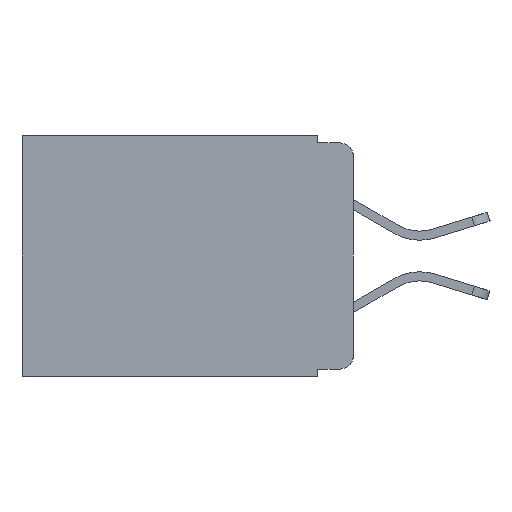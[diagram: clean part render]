
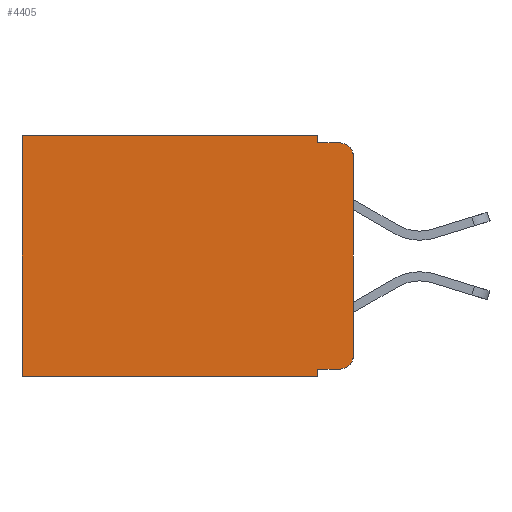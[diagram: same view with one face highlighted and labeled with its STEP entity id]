
A CAD part, left-side view. The second image highlights one B-rep face of the part: STEP entity #4405.
In plain terms, the highlighted planar face has unit normal (-1, 0, 0).
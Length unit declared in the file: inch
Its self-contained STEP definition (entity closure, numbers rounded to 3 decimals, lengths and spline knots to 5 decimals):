
#244 = VECTOR ( 'NONE', #6676, 39.37008 ) ;
#445 = VECTOR ( 'NONE', #9606, 39.37008 ) ;
#461 = ORIENTED_EDGE ( 'NONE', *, *, #2379, .T. ) ;
#706 = EDGE_LOOP ( 'NONE', ( #2293, #2764, #3546, #811, #461, #4432, #4359, #2546, #3100, #4057 ) ) ;
#811 = ORIENTED_EDGE ( 'NONE', *, *, #1928, .F. ) ;
#1293 = EDGE_CURVE ( 'NONE', #8706, #2113, #6968, .T. ) ;
#1497 = LINE ( 'NONE', #3207, #8030 ) ;
#1835 = EDGE_CURVE ( 'NONE', #3333, #5252, #5842, .T. ) ;
#1911 = EDGE_CURVE ( 'NONE', #3333, #3045, #3982, .T. ) ;
#1913 = EDGE_CURVE ( 'NONE', #5400, #3045, #1497, .T. ) ;
#1928 = EDGE_CURVE ( 'NONE', #6808, #5400, #9977, .T. ) ;
#1972 = EDGE_CURVE ( 'NONE', #2336, #2113, #5190, .T. ) ;
#1988 = EDGE_CURVE ( 'NONE', #3810, #8706, #2867, .T. ) ;
#2025 = EDGE_CURVE ( 'NONE', #3810, #10645, #6342, .T. ) ;
#2074 = EDGE_CURVE ( 'NONE', #10645, #5252, #3568, .T. ) ;
#2103 = CARTESIAN_POINT ( 'NONE',  ( 0.298, 0.051, -0.343 ) ) ;
#2113 = VERTEX_POINT ( 'NONE', #9554 ) ;
#2293 = ORIENTED_EDGE ( 'NONE', *, *, #1835, .F. ) ;
#2336 = VERTEX_POINT ( 'NONE', #8853 ) ;
#2379 = EDGE_CURVE ( 'NONE', #6808, #2336, #9163, .T. ) ;
#2443 = DIRECTION ( 'NONE',  ( -1., 0., 0. ) ) ;
#2546 = ORIENTED_EDGE ( 'NONE', *, *, #1988, .F. ) ;
#2573 = CARTESIAN_POINT ( 'NONE',  ( 0.298, 0.02, -0.313 ) ) ;
#2764 = ORIENTED_EDGE ( 'NONE', *, *, #1911, .T. ) ;
#2867 = LINE ( 'NONE', #8884, #7063 ) ;
#2917 = FACE_OUTER_BOUND ( 'NONE', #706, .T. ) ;
#3023 = CARTESIAN_POINT ( 'NONE',  ( 0.298, 0., 0. ) ) ;
#3045 = VERTEX_POINT ( 'NONE', #4628 ) ;
#3067 = CARTESIAN_POINT ( 'NONE',  ( 0.298, 0.02, -0.03 ) ) ;
#3100 = ORIENTED_EDGE ( 'NONE', *, *, #2025, .T. ) ;
#3207 = CARTESIAN_POINT ( 'NONE',  ( 0.298, 0.051, -0.01 ) ) ;
#3281 = VECTOR ( 'NONE', #9714, 39.37008 ) ;
#3333 = VERTEX_POINT ( 'NONE', #9575 ) ;
#3546 = ORIENTED_EDGE ( 'NONE', *, *, #1913, .F. ) ;
#3568 = CIRCLE ( 'NONE', #4679, 0.02 ) ;
#3810 = VERTEX_POINT ( 'NONE', #9074 ) ;
#3931 = CARTESIAN_POINT ( 'NONE',  ( 0.298, 0.051, 0. ) ) ;
#3982 = CIRCLE ( 'NONE', #9063, 0.02 ) ;
#4057 = ORIENTED_EDGE ( 'NONE', *, *, #2074, .T. ) ;
#4297 = DIRECTION ( 'NONE',  ( 0., 1., 0. ) ) ;
#4359 = ORIENTED_EDGE ( 'NONE', *, *, #1293, .F. ) ;
#4405 = ADVANCED_FACE ( 'NONE', ( #2917 ), #9055, .F. ) ;
#4432 = ORIENTED_EDGE ( 'NONE', *, *, #1972, .T. ) ;
#4542 = DIRECTION ( 'NONE',  ( 0., 0., -1. ) ) ;
#4552 = CARTESIAN_POINT ( 'NONE',  ( 0.298, 0.051, -0.333 ) ) ;
#4628 = CARTESIAN_POINT ( 'NONE',  ( 0.298, 0.02, -0.01 ) ) ;
#4679 = AXIS2_PLACEMENT_3D ( 'NONE', #2573, #2443, #7552 ) ;
#4767 = VECTOR ( 'NONE', #4297, 39.37008 ) ;
#4784 = CARTESIAN_POINT ( 'NONE',  ( 0.298, 0., 0. ) ) ;
#4799 = DIRECTION ( 'NONE',  ( -1., 0., 0. ) ) ;
#5028 = DIRECTION ( 'NONE',  ( 0., 0., -1. ) ) ;
#5190 = LINE ( 'NONE', #7516, #244 ) ;
#5252 = VERTEX_POINT ( 'NONE', #8470 ) ;
#5400 = VERTEX_POINT ( 'NONE', #7203 ) ;
#5533 = DIRECTION ( 'NONE',  ( 0., -1., 0. ) ) ;
#5842 = LINE ( 'NONE', #7781, #3281 ) ;
#6342 = LINE ( 'NONE', #4552, #10081 ) ;
#6513 = CARTESIAN_POINT ( 'NONE',  ( 0.298, 0.02, -0.333 ) ) ;
#6522 = DIRECTION ( 'NONE',  ( 0., -1., 0. ) ) ;
#6533 = CARTESIAN_POINT ( 'NONE',  ( 0.298, 0.051, 0. ) ) ;
#6676 = DIRECTION ( 'NONE',  ( 0., 0., -1. ) ) ;
#6808 = VERTEX_POINT ( 'NONE', #3931 ) ;
#6968 = LINE ( 'NONE', #7459, #445 ) ;
#7013 = AXIS2_PLACEMENT_3D ( 'NONE', #4784, #8979, #5028 ) ;
#7063 = VECTOR ( 'NONE', #8876, 39.37008 ) ;
#7203 = CARTESIAN_POINT ( 'NONE',  ( 0.298, 0.051, -0.01 ) ) ;
#7459 = CARTESIAN_POINT ( 'NONE',  ( 0.298, 0., -0.343 ) ) ;
#7516 = CARTESIAN_POINT ( 'NONE',  ( 0.298, 0.473, 0. ) ) ;
#7552 = DIRECTION ( 'NONE',  ( 0., 0., -1. ) ) ;
#7781 = CARTESIAN_POINT ( 'NONE',  ( 0.298, 0., 0. ) ) ;
#7788 = VECTOR ( 'NONE', #7940, 39.37008 ) ;
#7940 = DIRECTION ( 'NONE',  ( 0., 0., -1. ) ) ;
#8030 = VECTOR ( 'NONE', #5533, 39.37008 ) ;
#8470 = CARTESIAN_POINT ( 'NONE',  ( 0.298, 0., -0.313 ) ) ;
#8706 = VERTEX_POINT ( 'NONE', #2103 ) ;
#8853 = CARTESIAN_POINT ( 'NONE',  ( 0.298, 0.473, 0. ) ) ;
#8876 = DIRECTION ( 'NONE',  ( 0., 0., -1. ) ) ;
#8884 = CARTESIAN_POINT ( 'NONE',  ( 0.298, 0.051, 0. ) ) ;
#8979 = DIRECTION ( 'NONE',  ( 1., 0., 0. ) ) ;
#9055 = PLANE ( 'NONE',  #7013 ) ;
#9063 = AXIS2_PLACEMENT_3D ( 'NONE', #3067, #4799, #4542 ) ;
#9074 = CARTESIAN_POINT ( 'NONE',  ( 0.298, 0.051, -0.333 ) ) ;
#9163 = LINE ( 'NONE', #3023, #4767 ) ;
#9554 = CARTESIAN_POINT ( 'NONE',  ( 0.298, 0.473, -0.343 ) ) ;
#9575 = CARTESIAN_POINT ( 'NONE',  ( 0.298, 0., -0.03 ) ) ;
#9606 = DIRECTION ( 'NONE',  ( 0., 1., 0. ) ) ;
#9714 = DIRECTION ( 'NONE',  ( 0., 0., -1. ) ) ;
#9977 = LINE ( 'NONE', #6533, #7788 ) ;
#10081 = VECTOR ( 'NONE', #6522, 39.37008 ) ;
#10645 = VERTEX_POINT ( 'NONE', #6513 ) ;
